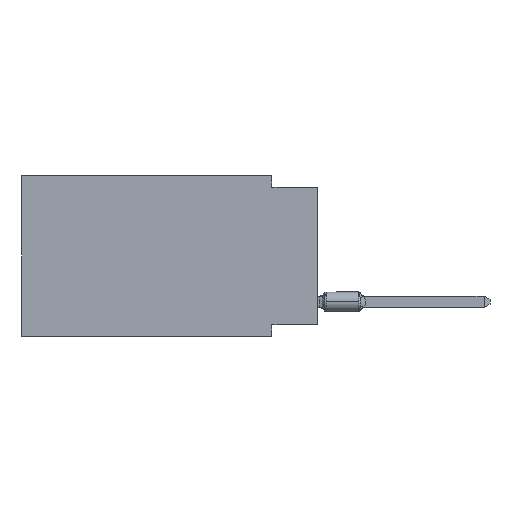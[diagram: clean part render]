
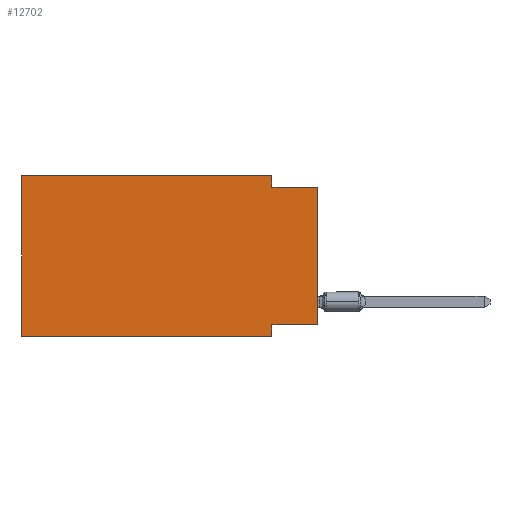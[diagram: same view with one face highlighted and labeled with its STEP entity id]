
A CAD part, left-side view. The second image highlights one B-rep face of the part: STEP entity #12702.
In plain terms, the highlighted planar face has unit normal (-1, 0, 0).
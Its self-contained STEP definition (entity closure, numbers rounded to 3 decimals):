
#57 = CARTESIAN_POINT ( 'NONE',  ( 0., 16.383, 0. ) ) ;
#140 = DIRECTION ( 'NONE',  ( 0., 0., 1. ) ) ;
#195 = CARTESIAN_POINT ( 'NONE',  ( 0., 0., 0. ) ) ;
#259 = VECTOR ( 'NONE', #140, 1000. ) ;
#354 = VERTEX_POINT ( 'NONE', #3163 ) ;
#392 = EDGE_CURVE ( 'NONE', #10967, #7937, #3583, .T. ) ;
#963 = VECTOR ( 'NONE', #16334, 1000. ) ;
#1290 = VECTOR ( 'NONE', #2777, 1000. ) ;
#1765 = ORIENTED_EDGE ( 'NONE', *, *, #7930, .T. ) ;
#1772 = CARTESIAN_POINT ( 'NONE',  ( 0., 2.54, 0. ) ) ;
#2676 = VECTOR ( 'NONE', #15768, 1000. ) ;
#2777 = DIRECTION ( 'NONE',  ( 0., -1., 0. ) ) ;
#2877 = FACE_OUTER_BOUND ( 'NONE', #2962, .T. ) ;
#2962 = EDGE_LOOP ( 'NONE', ( #1765, #13141, #7691, #4367, #13110, #11101, #11949, #12435 ) ) ;
#3163 = CARTESIAN_POINT ( 'NONE',  ( 0., 2.54, -8.89 ) ) ;
#3193 = LINE ( 'NONE', #3273, #2676 ) ;
#3273 = CARTESIAN_POINT ( 'NONE',  ( 0., 0., -0.635 ) ) ;
#3502 = CARTESIAN_POINT ( 'NONE',  ( 0., 16.383, 0. ) ) ;
#3583 = LINE ( 'NONE', #11161, #11502 ) ;
#3633 = VERTEX_POINT ( 'NONE', #1772 ) ;
#3681 = LINE ( 'NONE', #12976, #6984 ) ;
#3959 = CARTESIAN_POINT ( 'NONE',  ( 0., 16.383, 0. ) ) ;
#4367 = ORIENTED_EDGE ( 'NONE', *, *, #5083, .F. ) ;
#4896 = CARTESIAN_POINT ( 'NONE',  ( 0., 2.54, 0. ) ) ;
#5083 = EDGE_CURVE ( 'NONE', #9863, #3633, #14088, .T. ) ;
#6035 = VERTEX_POINT ( 'NONE', #7570 ) ;
#6068 = DIRECTION ( 'NONE',  ( 0., 0., -1. ) ) ;
#6478 = LINE ( 'NONE', #57, #259 ) ;
#6923 = VERTEX_POINT ( 'NONE', #7360 ) ;
#6984 = VECTOR ( 'NONE', #15414, 1000. ) ;
#6999 = EDGE_CURVE ( 'NONE', #7177, #354, #16244, .T. ) ;
#7107 = DIRECTION ( 'NONE',  ( 0., 1., 0. ) ) ;
#7177 = VERTEX_POINT ( 'NONE', #12125 ) ;
#7360 = CARTESIAN_POINT ( 'NONE',  ( 0., 2.54, -0.635 ) ) ;
#7483 = CARTESIAN_POINT ( 'NONE',  ( 0., 2.54, -8.255 ) ) ;
#7570 = CARTESIAN_POINT ( 'NONE',  ( 0., 0., -0.635 ) ) ;
#7657 = VECTOR ( 'NONE', #11511, 1000. ) ;
#7691 = ORIENTED_EDGE ( 'NONE', *, *, #12958, .F. ) ;
#7751 = DIRECTION ( 'NONE',  ( 0., 0., -1. ) ) ;
#7930 = EDGE_CURVE ( 'NONE', #10967, #6035, #11427, .T. ) ;
#7937 = VERTEX_POINT ( 'NONE', #7483 ) ;
#9863 = VERTEX_POINT ( 'NONE', #3502 ) ;
#9884 = CARTESIAN_POINT ( 'NONE',  ( 0., 16.383, -8.89 ) ) ;
#9897 = AXIS2_PLACEMENT_3D ( 'NONE', #3959, #12859, #7751 ) ;
#9911 = VECTOR ( 'NONE', #6068, 1000. ) ;
#10271 = PLANE ( 'NONE',  #9897 ) ;
#10967 = VERTEX_POINT ( 'NONE', #14479 ) ;
#11101 = ORIENTED_EDGE ( 'NONE', *, *, #6999, .T. ) ;
#11161 = CARTESIAN_POINT ( 'NONE',  ( 0., 0., -8.255 ) ) ;
#11427 = LINE ( 'NONE', #195, #7657 ) ;
#11502 = VECTOR ( 'NONE', #7107, 1000. ) ;
#11511 = DIRECTION ( 'NONE',  ( 0., 0., 1. ) ) ;
#11675 = CARTESIAN_POINT ( 'NONE',  ( 0., 16.383, 0. ) ) ;
#11949 = ORIENTED_EDGE ( 'NONE', *, *, #12178, .F. ) ;
#12125 = CARTESIAN_POINT ( 'NONE',  ( 0., 16.383, -8.89 ) ) ;
#12178 = EDGE_CURVE ( 'NONE', #7937, #354, #3681, .T. ) ;
#12435 = ORIENTED_EDGE ( 'NONE', *, *, #392, .F. ) ;
#12667 = EDGE_CURVE ( 'NONE', #7177, #9863, #6478, .T. ) ;
#12702 = ADVANCED_FACE ( 'NONE', ( #2877 ), #10271, .F. ) ;
#12859 = DIRECTION ( 'NONE',  ( 1., 0., 0. ) ) ;
#12958 = EDGE_CURVE ( 'NONE', #3633, #6923, #16382, .T. ) ;
#12976 = CARTESIAN_POINT ( 'NONE',  ( 0., 2.54, -8.89 ) ) ;
#13110 = ORIENTED_EDGE ( 'NONE', *, *, #12667, .F. ) ;
#13141 = ORIENTED_EDGE ( 'NONE', *, *, #13143, .F. ) ;
#13143 = EDGE_CURVE ( 'NONE', #6923, #6035, #3193, .T. ) ;
#14088 = LINE ( 'NONE', #11675, #1290 ) ;
#14479 = CARTESIAN_POINT ( 'NONE',  ( 0., 0., -8.255 ) ) ;
#15414 = DIRECTION ( 'NONE',  ( 0., 0., -1. ) ) ;
#15768 = DIRECTION ( 'NONE',  ( 0., -1., 0. ) ) ;
#16244 = LINE ( 'NONE', #9884, #963 ) ;
#16334 = DIRECTION ( 'NONE',  ( 0., -1., 0. ) ) ;
#16382 = LINE ( 'NONE', #4896, #9911 ) ;
